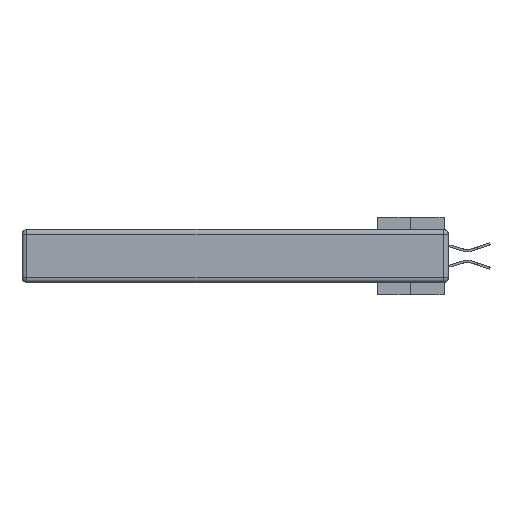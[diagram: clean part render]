
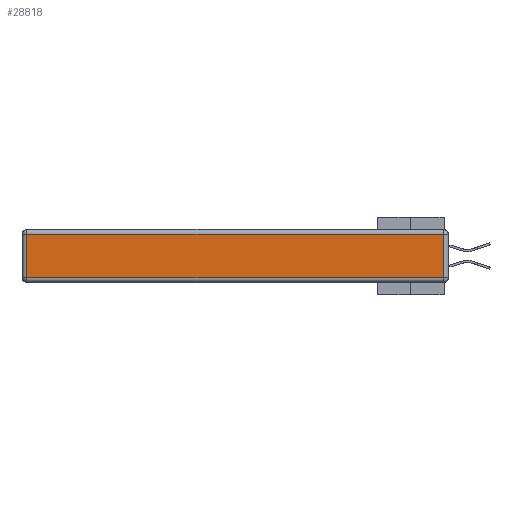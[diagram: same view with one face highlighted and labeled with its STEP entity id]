
A CAD part, left-side view. The second image highlights one B-rep face of the part: STEP entity #28818.
In plain terms, the highlighted planar face has unit normal (-1, 0, 0).
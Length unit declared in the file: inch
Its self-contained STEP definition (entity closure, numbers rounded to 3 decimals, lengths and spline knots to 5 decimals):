
#477 = CARTESIAN_POINT ( 'NONE',  ( 0., 0., -0.313 ) ) ;
#1419 = VERTEX_POINT ( 'NONE', #10521 ) ;
#1797 = EDGE_CURVE ( 'NONE', #20624, #17642, #38737, .T. ) ;
#3439 = EDGE_CURVE ( 'NONE', #35023, #20624, #11029, .T. ) ;
#7751 = CARTESIAN_POINT ( 'NONE',  ( 0., 2.72, -0.313 ) ) ;
#7954 = ORIENTED_EDGE ( 'NONE', *, *, #17490, .T. ) ;
#9251 = VECTOR ( 'NONE', #26662, 39.37008 ) ;
#9695 = ORIENTED_EDGE ( 'NONE', *, *, #13491, .T. ) ;
#10521 = CARTESIAN_POINT ( 'NONE',  ( 0., 0.03, -0.03 ) ) ;
#10522 = VECTOR ( 'NONE', #35355, 39.37008 ) ;
#11029 = LINE ( 'NONE', #15156, #10522 ) ;
#13411 = CARTESIAN_POINT ( 'NONE',  ( 0., 0.03, -0.313 ) ) ;
#13491 = EDGE_CURVE ( 'NONE', #1419, #35023, #22484, .T. ) ;
#13564 = VECTOR ( 'NONE', #29986, 39.37008 ) ;
#15156 = CARTESIAN_POINT ( 'NONE',  ( 0., 2.72, -0.343 ) ) ;
#17069 = ORIENTED_EDGE ( 'NONE', *, *, #3439, .T. ) ;
#17490 = EDGE_CURVE ( 'NONE', #17642, #1419, #39528, .T. ) ;
#17642 = VERTEX_POINT ( 'NONE', #13411 ) ;
#19548 = CARTESIAN_POINT ( 'NONE',  ( 0., 2.75, -0.03 ) ) ;
#20287 = FACE_OUTER_BOUND ( 'NONE', #36796, .T. ) ;
#20624 = VERTEX_POINT ( 'NONE', #7751 ) ;
#22484 = LINE ( 'NONE', #19548, #13564 ) ;
#24603 = PLANE ( 'NONE',  #37469 ) ;
#26662 = DIRECTION ( 'NONE',  ( 0., 0., 1. ) ) ;
#27582 = CARTESIAN_POINT ( 'NONE',  ( 0., 2.72, -0.03 ) ) ;
#27623 = DIRECTION ( 'NONE',  ( 0., -1., 0. ) ) ;
#28818 = ADVANCED_FACE ( 'NONE', ( #20287 ), #24603, .T. ) ;
#29986 = DIRECTION ( 'NONE',  ( 0., 1., 0. ) ) ;
#33944 = ORIENTED_EDGE ( 'NONE', *, *, #1797, .T. ) ;
#35023 = VERTEX_POINT ( 'NONE', #27582 ) ;
#35050 = DIRECTION ( 'NONE',  ( -1., 0., 0. ) ) ;
#35209 = CARTESIAN_POINT ( 'NONE',  ( 0., 0., -0.343 ) ) ;
#35355 = DIRECTION ( 'NONE',  ( 0., 0., -1. ) ) ;
#35932 = DIRECTION ( 'NONE',  ( 0., 0., 1. ) ) ;
#36796 = EDGE_LOOP ( 'NONE', ( #33944, #7954, #9695, #17069 ) ) ;
#37469 = AXIS2_PLACEMENT_3D ( 'NONE', #35209, #35050, #35932 ) ;
#38202 = VECTOR ( 'NONE', #27623, 39.37008 ) ;
#38737 = LINE ( 'NONE', #477, #38202 ) ;
#39528 = LINE ( 'NONE', #40263, #9251 ) ;
#40263 = CARTESIAN_POINT ( 'NONE',  ( 0., 0.03, -0.343 ) ) ;
